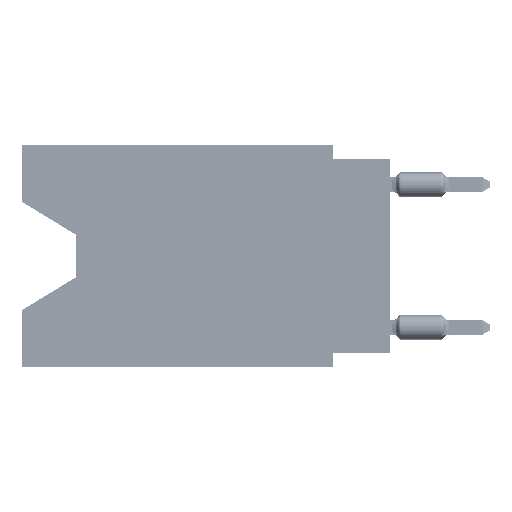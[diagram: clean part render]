
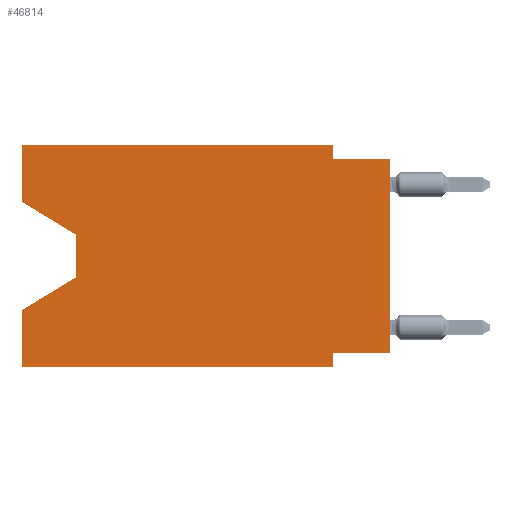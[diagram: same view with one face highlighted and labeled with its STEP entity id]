
A CAD part, left-side view. The second image highlights one B-rep face of the part: STEP entity #46814.
In plain terms, the highlighted planar face has unit normal (-1, 0, 0).
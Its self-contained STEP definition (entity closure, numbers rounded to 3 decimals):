
#549 = CARTESIAN_POINT ( 'NONE',  ( 0., 16.383, 0. ) ) ;
#627 = VECTOR ( 'NONE', #33310, 1000. ) ;
#1128 = ORIENTED_EDGE ( 'NONE', *, *, #54254, .F. ) ;
#1400 = FACE_OUTER_BOUND ( 'NONE', #47694, .T. ) ;
#1507 = DIRECTION ( 'NONE',  ( 0., 0., 1. ) ) ;
#1685 = VERTEX_POINT ( 'NONE', #3290 ) ;
#2992 = VECTOR ( 'NONE', #1507, 1000. ) ;
#3290 = CARTESIAN_POINT ( 'NONE',  ( 0., 2.54, -0.635 ) ) ;
#3751 = CARTESIAN_POINT ( 'NONE',  ( 0., 16.383, -2.546 ) ) ;
#4486 = ORIENTED_EDGE ( 'NONE', *, *, #54161, .T. ) ;
#4569 = ORIENTED_EDGE ( 'NONE', *, *, #51263, .T. ) ;
#5112 = DIRECTION ( 'NONE',  ( 0., 0., -1. ) ) ;
#5634 = VERTEX_POINT ( 'NONE', #20912 ) ;
#5832 = VERTEX_POINT ( 'NONE', #55230 ) ;
#6061 = VECTOR ( 'NONE', #43386, 1000. ) ;
#6424 = VERTEX_POINT ( 'NONE', #20775 ) ;
#6950 = DIRECTION ( 'NONE',  ( 0., -1., 0. ) ) ;
#7251 = LINE ( 'NONE', #51116, #32463 ) ;
#7386 = VERTEX_POINT ( 'NONE', #36576 ) ;
#7544 = LINE ( 'NONE', #56537, #31077 ) ;
#8128 = LINE ( 'NONE', #56261, #6061 ) ;
#8544 = VECTOR ( 'NONE', #21223, 1000. ) ;
#9009 = EDGE_CURVE ( 'NONE', #5634, #51830, #44317, .T. ) ;
#9991 = DIRECTION ( 'NONE',  ( 0., -1., 0. ) ) ;
#10341 = CARTESIAN_POINT ( 'NONE',  ( 0., 16.383, -2.546 ) ) ;
#10740 = CARTESIAN_POINT ( 'NONE',  ( 0., 13.97, -4.013 ) ) ;
#11373 = VECTOR ( 'NONE', #54586, 1000. ) ;
#12338 = LINE ( 'NONE', #3751, #8544 ) ;
#12353 = CARTESIAN_POINT ( 'NONE',  ( 0., 2.54, -9.271 ) ) ;
#12912 = EDGE_CURVE ( 'NONE', #54451, #51041, #7251, .T. ) ;
#13040 = CARTESIAN_POINT ( 'NONE',  ( 0., 2.54, -9.906 ) ) ;
#13280 = ORIENTED_EDGE ( 'NONE', *, *, #48520, .F. ) ;
#13551 = DIRECTION ( 'NONE',  ( 0., 0.855, -0.519 ) ) ;
#13925 = CARTESIAN_POINT ( 'NONE',  ( 0., 16.383, 0. ) ) ;
#18143 = CARTESIAN_POINT ( 'NONE',  ( 0., 0., -9.271 ) ) ;
#18903 = ORIENTED_EDGE ( 'NONE', *, *, #55326, .F. ) ;
#18981 = CARTESIAN_POINT ( 'NONE',  ( 0., 0., 0. ) ) ;
#19465 = CARTESIAN_POINT ( 'NONE',  ( 0., 2.54, 0. ) ) ;
#20775 = CARTESIAN_POINT ( 'NONE',  ( 0., 13.97, -4.013 ) ) ;
#20909 = ORIENTED_EDGE ( 'NONE', *, *, #47321, .T. ) ;
#20912 = CARTESIAN_POINT ( 'NONE',  ( 0., 16.383, 0. ) ) ;
#21016 = LINE ( 'NONE', #18981, #2992 ) ;
#21223 = DIRECTION ( 'NONE',  ( 0., -0.855, -0.519 ) ) ;
#21862 = DIRECTION ( 'NONE',  ( 0., 0., 1. ) ) ;
#22146 = CARTESIAN_POINT ( 'NONE',  ( 0., 16.383, -7.36 ) ) ;
#23735 = CARTESIAN_POINT ( 'NONE',  ( 0., 0., -0.635 ) ) ;
#24017 = LINE ( 'NONE', #23735, #41941 ) ;
#24443 = VECTOR ( 'NONE', #6950, 1000. ) ;
#24990 = CARTESIAN_POINT ( 'NONE',  ( 0., 16.383, 0. ) ) ;
#25489 = VERTEX_POINT ( 'NONE', #10341 ) ;
#26507 = VERTEX_POINT ( 'NONE', #22146 ) ;
#26517 = EDGE_CURVE ( 'NONE', #37787, #26507, #47955, .T. ) ;
#26579 = VECTOR ( 'NONE', #53739, 1000. ) ;
#26685 = ORIENTED_EDGE ( 'NONE', *, *, #38923, .T. ) ;
#27835 = ORIENTED_EDGE ( 'NONE', *, *, #26517, .F. ) ;
#28709 = CARTESIAN_POINT ( 'NONE',  ( 0., 13.97, -5.893 ) ) ;
#28735 = CARTESIAN_POINT ( 'NONE',  ( 0., 16.383, -9.906 ) ) ;
#29029 = DIRECTION ( 'NONE',  ( 0., 0., -1. ) ) ;
#29061 = LINE ( 'NONE', #10740, #11373 ) ;
#29279 = LINE ( 'NONE', #24990, #627 ) ;
#31077 = VECTOR ( 'NONE', #13551, 1000. ) ;
#31215 = ORIENTED_EDGE ( 'NONE', *, *, #9009, .F. ) ;
#32463 = VECTOR ( 'NONE', #29029, 1000. ) ;
#32762 = LINE ( 'NONE', #28735, #24443 ) ;
#33310 = DIRECTION ( 'NONE',  ( 0., 0., 1. ) ) ;
#35965 = VECTOR ( 'NONE', #21862, 1000. ) ;
#36034 = VERTEX_POINT ( 'NONE', #28709 ) ;
#36576 = CARTESIAN_POINT ( 'NONE',  ( 0., 0., -9.271 ) ) ;
#36621 = ORIENTED_EDGE ( 'NONE', *, *, #40083, .T. ) ;
#37787 = VERTEX_POINT ( 'NONE', #39273 ) ;
#38923 = EDGE_CURVE ( 'NONE', #25489, #6424, #12338, .T. ) ;
#39273 = CARTESIAN_POINT ( 'NONE',  ( 0., 16.383, -9.906 ) ) ;
#40083 = EDGE_CURVE ( 'NONE', #7386, #5832, #21016, .T. ) ;
#40941 = PLANE ( 'NONE',  #52547 ) ;
#41941 = VECTOR ( 'NONE', #9991, 1000. ) ;
#43386 = DIRECTION ( 'NONE',  ( 0., 0., -1. ) ) ;
#43642 = CARTESIAN_POINT ( 'NONE',  ( 0., 16.383, 0. ) ) ;
#44227 = LINE ( 'NONE', #18143, #50053 ) ;
#44317 = LINE ( 'NONE', #13925, #26579 ) ;
#44392 = DIRECTION ( 'NONE',  ( 1., 0., 0. ) ) ;
#46814 = ADVANCED_FACE ( 'NONE', ( #1400 ), #40941, .F. ) ;
#47321 = EDGE_CURVE ( 'NONE', #6424, #36034, #29061, .T. ) ;
#47694 = EDGE_LOOP ( 'NONE', ( #26685, #20909, #4486, #27835, #4569, #52620, #1128, #36621, #51865, #18903, #31215, #13280 ) ) ;
#47955 = LINE ( 'NONE', #43642, #35965 ) ;
#48520 = EDGE_CURVE ( 'NONE', #25489, #5634, #29279, .T. ) ;
#50053 = VECTOR ( 'NONE', #52817, 1000. ) ;
#50289 = EDGE_CURVE ( 'NONE', #1685, #5832, #24017, .T. ) ;
#51041 = VERTEX_POINT ( 'NONE', #13040 ) ;
#51116 = CARTESIAN_POINT ( 'NONE',  ( 0., 2.54, -9.906 ) ) ;
#51263 = EDGE_CURVE ( 'NONE', #37787, #51041, #32762, .T. ) ;
#51830 = VERTEX_POINT ( 'NONE', #19465 ) ;
#51865 = ORIENTED_EDGE ( 'NONE', *, *, #50289, .F. ) ;
#52547 = AXIS2_PLACEMENT_3D ( 'NONE', #549, #44392, #5112 ) ;
#52620 = ORIENTED_EDGE ( 'NONE', *, *, #12912, .F. ) ;
#52817 = DIRECTION ( 'NONE',  ( 0., 1., 0. ) ) ;
#53739 = DIRECTION ( 'NONE',  ( 0., -1., 0. ) ) ;
#54161 = EDGE_CURVE ( 'NONE', #36034, #26507, #7544, .T. ) ;
#54254 = EDGE_CURVE ( 'NONE', #7386, #54451, #44227, .T. ) ;
#54451 = VERTEX_POINT ( 'NONE', #12353 ) ;
#54586 = DIRECTION ( 'NONE',  ( 0., 0., -1. ) ) ;
#55230 = CARTESIAN_POINT ( 'NONE',  ( 0., 0., -0.635 ) ) ;
#55326 = EDGE_CURVE ( 'NONE', #51830, #1685, #8128, .T. ) ;
#56261 = CARTESIAN_POINT ( 'NONE',  ( 0., 2.54, 0. ) ) ;
#56537 = CARTESIAN_POINT ( 'NONE',  ( 0., 13.97, -5.893 ) ) ;
